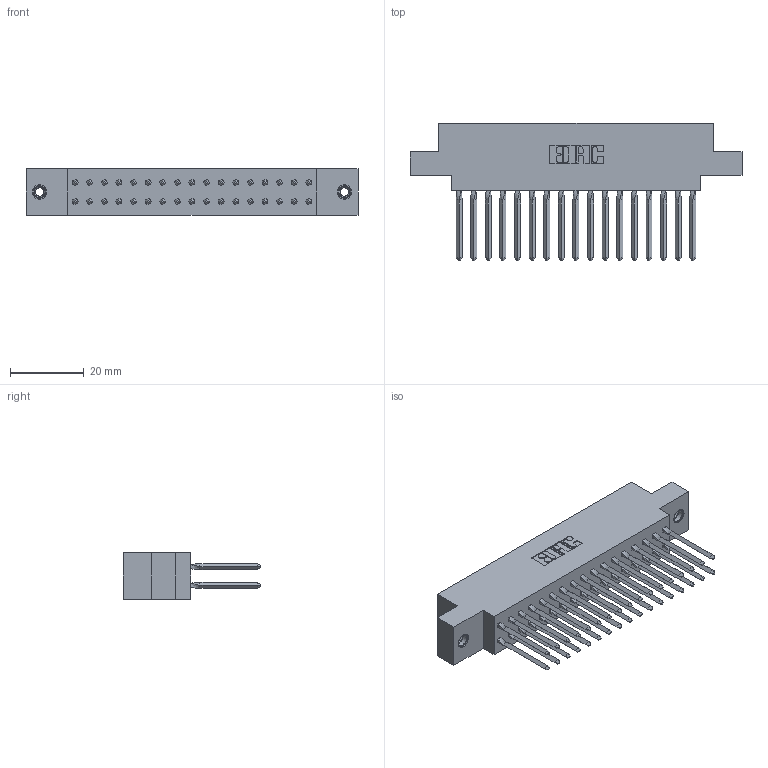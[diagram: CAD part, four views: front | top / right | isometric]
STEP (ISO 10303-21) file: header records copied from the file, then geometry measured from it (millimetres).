
FILE_DESCRIPTION (( 'STEP AP203' ), '1' );
FILE_NAME ('317-034-542-878.STEP', '2020-02-27T22:05:40', ( '' ), ( '' ), 'SwSTEP 2.0', 'SolidWorks 2016', '' );
FILE_SCHEMA (( 'CONFIG_CONTROL_DESIGN' ));
Length unit declared in the file: inch
Products named in the file (4): 317 Part_.156 Dia - TI; 317-034-542-878; 345-250-001_345-250-003-102; 317-290-003_542
Assembly tree (37 placements, depth 2):
  317-034-542-878
    317 Part_.156 Dia - TI
    317-290-003_542  x34
    345-250-001_345-250-003-102  x2
Bounding box: 90.07 x 37.34 x 12.7 mm (x, y, z)
Volume: 13951.8 mm3; surface area: 18621.6 mm2
Topology: 37 solids, 37 shells, 2100 faces, 5851 edges, 3734 vertices
Faces by surface type: plane 1654, cylinder 294, bspline 136, cone 12, torus 4
Entity records: 28264 total; most frequent: CARTESIAN_POINT 5148, ORIENTED_EDGE 4804, DIRECTION 4124, EDGE_CURVE 2402, VECTOR 2212, LINE 2212, VERTEX_POINT 1592, AXIS2_PLACEMENT_3D 956
